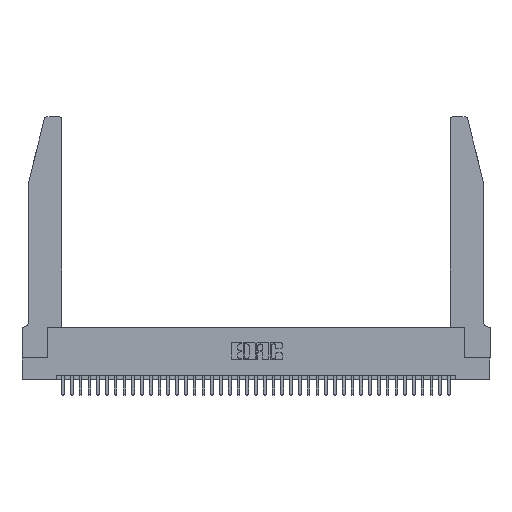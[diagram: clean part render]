
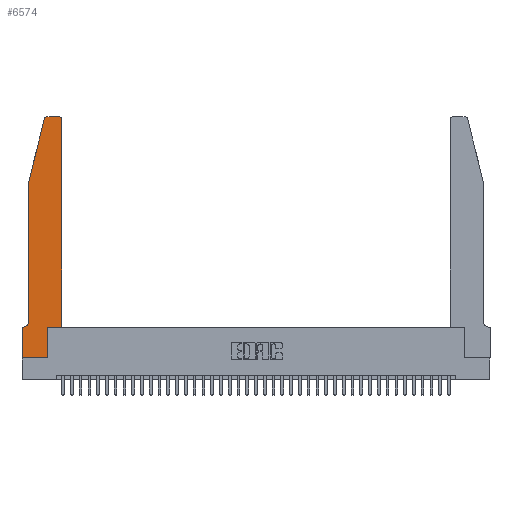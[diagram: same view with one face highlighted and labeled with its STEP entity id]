
A CAD part, top view. The second image highlights one B-rep face of the part: STEP entity #6574.
In plain terms, the highlighted planar face has unit normal (0, 0, 1).
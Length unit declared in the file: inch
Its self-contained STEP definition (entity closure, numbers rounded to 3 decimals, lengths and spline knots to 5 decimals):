
#634 = EDGE_CURVE ( 'NONE', #37947, #3032, #37487, .T. ) ;
#2726 = VECTOR ( 'NONE', #35909, 39.37008 ) ;
#2989 = DIRECTION ( 'NONE',  ( -1., 0., 0. ) ) ;
#3001 = CARTESIAN_POINT ( 'NONE',  ( 0.4205, 2.75, 0.37 ) ) ;
#3032 = VERTEX_POINT ( 'NONE', #34089 ) ;
#3548 = CARTESIAN_POINT ( 'NONE',  ( 0., 0., 0.37 ) ) ;
#3642 = PLANE ( 'NONE',  #33343 ) ;
#4158 = CARTESIAN_POINT ( 'NONE',  ( 0.4505, 0.35, 0.37 ) ) ;
#5304 = ORIENTED_EDGE ( 'NONE', *, *, #8775, .T. ) ;
#5938 = VECTOR ( 'NONE', #6540, 39.37008 ) ;
#6540 = DIRECTION ( 'NONE',  ( 1., 0., 0. ) ) ;
#6574 = ADVANCED_FACE ( 'NONE', ( #28394 ), #3642, .T. ) ;
#6765 = DIRECTION ( 'NONE',  ( 0., 0., 1. ) ) ;
#6960 = VECTOR ( 'NONE', #2989, 39.37008 ) ;
#6967 = CIRCLE ( 'NONE', #15524, 0.03 ) ;
#7053 = CARTESIAN_POINT ( 'NONE',  ( 0.0055, 0.35, 0.37 ) ) ;
#7141 = CARTESIAN_POINT ( 'NONE',  ( 0.0755, 0.42, 0.37 ) ) ;
#7703 = DIRECTION ( 'NONE',  ( 0., 0., 1. ) ) ;
#8132 = VECTOR ( 'NONE', #22174, 39.37008 ) ;
#8473 = EDGE_CURVE ( 'NONE', #11708, #22744, #28240, .T. ) ;
#8633 = CARTESIAN_POINT ( 'NONE',  ( 0.0755, 2., 0.37 ) ) ;
#8764 = EDGE_CURVE ( 'NONE', #22744, #17480, #33547, .T. ) ;
#8775 = EDGE_CURVE ( 'NONE', #3032, #24623, #9099, .T. ) ;
#9099 = LINE ( 'NONE', #19075, #8132 ) ;
#10746 = ORIENTED_EDGE ( 'NONE', *, *, #20922, .T. ) ;
#11097 = VERTEX_POINT ( 'NONE', #19637 ) ;
#11151 = ORIENTED_EDGE ( 'NONE', *, *, #27052, .T. ) ;
#11708 = VERTEX_POINT ( 'NONE', #7053 ) ;
#12331 = DIRECTION ( 'NONE',  ( 0., 0., -1. ) ) ;
#12613 = CARTESIAN_POINT ( 'NONE',  ( 0., 0., 0.37 ) ) ;
#13115 = VECTOR ( 'NONE', #13272, 39.37008 ) ;
#13272 = DIRECTION ( 'NONE',  ( 0., 1., 0. ) ) ;
#13324 = CARTESIAN_POINT ( 'NONE',  ( 0.4505, 0.35, 0.37 ) ) ;
#13652 = CARTESIAN_POINT ( 'NONE',  ( 0.2865, 0., 0.37 ) ) ;
#15021 = AXIS2_PLACEMENT_3D ( 'NONE', #30669, #12331, #33745 ) ;
#15116 = VERTEX_POINT ( 'NONE', #8633 ) ;
#15184 = CIRCLE ( 'NONE', #15021, 0.07 ) ;
#15524 = AXIS2_PLACEMENT_3D ( 'NONE', #15639, #37005, #18738 ) ;
#15639 = CARTESIAN_POINT ( 'NONE',  ( 0.284, 2.72, 0.37 ) ) ;
#16280 = CARTESIAN_POINT ( 'NONE',  ( 0.0755, 2., 0.37 ) ) ;
#17160 = VECTOR ( 'NONE', #19366, 39.37008 ) ;
#17309 = VECTOR ( 'NONE', #25102, 39.37008 ) ;
#17480 = VERTEX_POINT ( 'NONE', #39152 ) ;
#17565 = VERTEX_POINT ( 'NONE', #39675 ) ;
#17643 = CIRCLE ( 'NONE', #36208, 0.03 ) ;
#18738 = DIRECTION ( 'NONE',  ( 1., 0., 0. ) ) ;
#19075 = CARTESIAN_POINT ( 'NONE',  ( 0.4505, 0.35, 0.37 ) ) ;
#19366 = DIRECTION ( 'NONE',  ( -0.239, -0.971, 0. ) ) ;
#19369 = CARTESIAN_POINT ( 'NONE',  ( 0.0755, 2., 0.37 ) ) ;
#19537 = VERTEX_POINT ( 'NONE', #28339 ) ;
#19637 = CARTESIAN_POINT ( 'NONE',  ( 0.4505, 2.72, 0.37 ) ) ;
#20922 = EDGE_CURVE ( 'NONE', #11097, #35762, #17643, .T. ) ;
#21069 = ORIENTED_EDGE ( 'NONE', *, *, #34628, .T. ) ;
#22174 = DIRECTION ( 'NONE',  ( 1., 0., 0. ) ) ;
#22435 = EDGE_CURVE ( 'NONE', #15116, #39776, #39002, .T. ) ;
#22744 = VERTEX_POINT ( 'NONE', #39075 ) ;
#23299 = LINE ( 'NONE', #12613, #5938 ) ;
#23364 = LINE ( 'NONE', #39726, #6960 ) ;
#24623 = VERTEX_POINT ( 'NONE', #4158 ) ;
#25102 = DIRECTION ( 'NONE',  ( 0., -1., 0. ) ) ;
#25668 = ORIENTED_EDGE ( 'NONE', *, *, #22435, .T. ) ;
#26107 = CARTESIAN_POINT ( 'NONE',  ( 0.4205, 2.72, 0.37 ) ) ;
#26419 = LINE ( 'NONE', #13324, #33564 ) ;
#27052 = EDGE_CURVE ( 'NONE', #24623, #11097, #26419, .T. ) ;
#28240 = LINE ( 'NONE', #36045, #2726 ) ;
#28249 = DIRECTION ( 'NONE',  ( 1., 0., 0. ) ) ;
#28339 = CARTESIAN_POINT ( 'NONE',  ( 0.284, 2.75, 0.37 ) ) ;
#28362 = ORIENTED_EDGE ( 'NONE', *, *, #634, .T. ) ;
#28394 = FACE_OUTER_BOUND ( 'NONE', #33300, .T. ) ;
#28654 = CARTESIAN_POINT ( 'NONE',  ( 0.2865, 0.35, 0.37 ) ) ;
#28743 = ORIENTED_EDGE ( 'NONE', *, *, #33878, .T. ) ;
#29157 = DIRECTION ( 'NONE',  ( 1., 0., 0. ) ) ;
#29937 = VECTOR ( 'NONE', #34582, 39.37008 ) ;
#30669 = CARTESIAN_POINT ( 'NONE',  ( 0.0055, 0.42, 0.37 ) ) ;
#31060 = EDGE_CURVE ( 'NONE', #17480, #37947, #23299, .T. ) ;
#33300 = EDGE_LOOP ( 'NONE', ( #34472, #21069, #34595, #25668, #28743, #37692, #38047, #33380, #28362, #5304, #11151, #10746 ) ) ;
#33343 = AXIS2_PLACEMENT_3D ( 'NONE', #37293, #6765, #28249 ) ;
#33356 = EDGE_CURVE ( 'NONE', #17565, #15116, #34350, .T. ) ;
#33380 = ORIENTED_EDGE ( 'NONE', *, *, #31060, .T. ) ;
#33547 = LINE ( 'NONE', #3548, #17309 ) ;
#33564 = VECTOR ( 'NONE', #37763, 39.37008 ) ;
#33745 = DIRECTION ( 'NONE',  ( -1., 0., 0. ) ) ;
#33876 = EDGE_CURVE ( 'NONE', #35762, #19537, #23364, .T. ) ;
#33878 = EDGE_CURVE ( 'NONE', #39776, #11708, #15184, .T. ) ;
#34089 = CARTESIAN_POINT ( 'NONE',  ( 0.2865, 0.35, 0.37 ) ) ;
#34350 = LINE ( 'NONE', #16280, #17160 ) ;
#34472 = ORIENTED_EDGE ( 'NONE', *, *, #33876, .T. ) ;
#34582 = DIRECTION ( 'NONE',  ( 0., -1., 0. ) ) ;
#34595 = ORIENTED_EDGE ( 'NONE', *, *, #33356, .T. ) ;
#34628 = EDGE_CURVE ( 'NONE', #19537, #17565, #6967, .T. ) ;
#35762 = VERTEX_POINT ( 'NONE', #3001 ) ;
#35909 = DIRECTION ( 'NONE',  ( -1., 0., 0. ) ) ;
#36045 = CARTESIAN_POINT ( 'NONE',  ( 0.0755, 0.35, 0.37 ) ) ;
#36208 = AXIS2_PLACEMENT_3D ( 'NONE', #26107, #7703, #29157 ) ;
#37005 = DIRECTION ( 'NONE',  ( 0., 0., 1. ) ) ;
#37293 = CARTESIAN_POINT ( 'NONE',  ( 0., 0.35, 0.37 ) ) ;
#37487 = LINE ( 'NONE', #28654, #13115 ) ;
#37692 = ORIENTED_EDGE ( 'NONE', *, *, #8473, .T. ) ;
#37763 = DIRECTION ( 'NONE',  ( 0., 1., 0. ) ) ;
#37947 = VERTEX_POINT ( 'NONE', #13652 ) ;
#38047 = ORIENTED_EDGE ( 'NONE', *, *, #8764, .T. ) ;
#39002 = LINE ( 'NONE', #19369, #29937 ) ;
#39075 = CARTESIAN_POINT ( 'NONE',  ( 0., 0.35, 0.37 ) ) ;
#39152 = CARTESIAN_POINT ( 'NONE',  ( 0., 0., 0.37 ) ) ;
#39675 = CARTESIAN_POINT ( 'NONE',  ( 0.25487, 2.72718, 0.37 ) ) ;
#39726 = CARTESIAN_POINT ( 'NONE',  ( 0.2605, 2.75, 0.37 ) ) ;
#39776 = VERTEX_POINT ( 'NONE', #7141 ) ;
